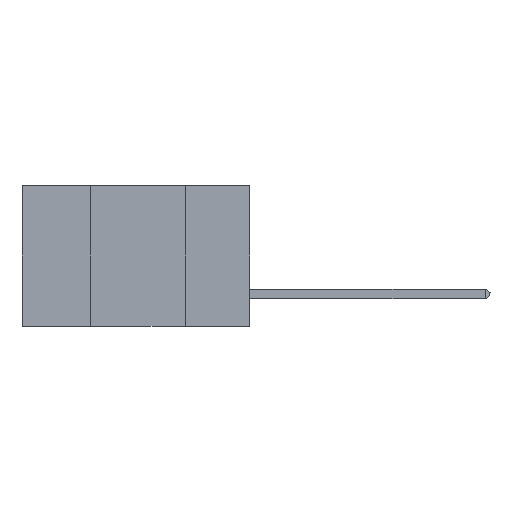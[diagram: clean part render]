
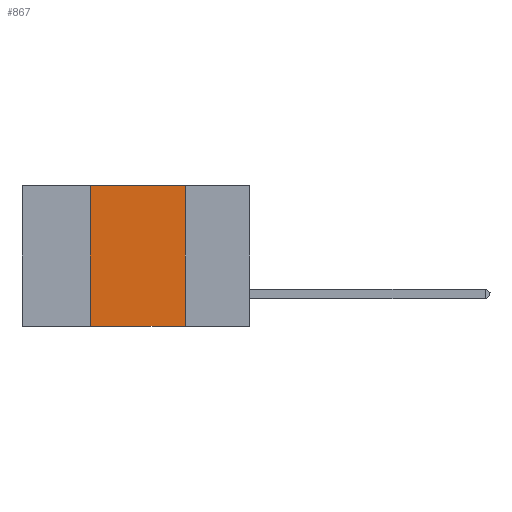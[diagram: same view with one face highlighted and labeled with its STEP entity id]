
A CAD part, left-side view. The second image highlights one B-rep face of the part: STEP entity #867.
In plain terms, the highlighted planar face has unit normal (-1, 0, 0).
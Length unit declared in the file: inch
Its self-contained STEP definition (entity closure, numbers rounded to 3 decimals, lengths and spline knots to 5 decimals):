
#100 = VECTOR ( 'NONE', #4592, 39.37008 ) ;
#669 = DIRECTION ( 'NONE',  ( 0., 0., -1. ) ) ;
#867 = ADVANCED_FACE ( 'NONE', ( #1939 ), #8767, .F. ) ;
#1110 = EDGE_CURVE ( 'NONE', #10636, #9905, #13705, .T. ) ;
#1291 = VERTEX_POINT ( 'NONE', #4663 ) ;
#1894 = ORIENTED_EDGE ( 'NONE', *, *, #5436, .F. ) ;
#1939 = FACE_OUTER_BOUND ( 'NONE', #13257, .T. ) ;
#3651 = CARTESIAN_POINT ( 'NONE',  ( 0., 0.17, 0. ) ) ;
#3675 = ORIENTED_EDGE ( 'NONE', *, *, #1110, .F. ) ;
#3711 = EDGE_CURVE ( 'NONE', #10761, #1291, #13244, .T. ) ;
#4373 = DIRECTION ( 'NONE',  ( 0., 0., -1. ) ) ;
#4592 = DIRECTION ( 'NONE',  ( 0., -1., 0. ) ) ;
#4663 = CARTESIAN_POINT ( 'NONE',  ( 0., 0.17, -0.37 ) ) ;
#5418 = DIRECTION ( 'NONE',  ( 1., 0., 0. ) ) ;
#5436 = EDGE_CURVE ( 'NONE', #9905, #10761, #8545, .T. ) ;
#5582 = ORIENTED_EDGE ( 'NONE', *, *, #3711, .F. ) ;
#5918 = VECTOR ( 'NONE', #12029, 39.37008 ) ;
#6578 = CARTESIAN_POINT ( 'NONE',  ( 0., 0.42, 0. ) ) ;
#6890 = LINE ( 'NONE', #13391, #100 ) ;
#7086 = VECTOR ( 'NONE', #14372, 39.37008 ) ;
#7927 = ORIENTED_EDGE ( 'NONE', *, *, #8289, .T. ) ;
#8289 = EDGE_CURVE ( 'NONE', #10636, #1291, #6890, .T. ) ;
#8545 = LINE ( 'NONE', #10694, #5918 ) ;
#8767 = PLANE ( 'NONE',  #14174 ) ;
#8982 = CARTESIAN_POINT ( 'NONE',  ( 0., 0.42, 0. ) ) ;
#9905 = VERTEX_POINT ( 'NONE', #8982 ) ;
#10473 = VECTOR ( 'NONE', #669, 39.37008 ) ;
#10636 = VERTEX_POINT ( 'NONE', #11184 ) ;
#10694 = CARTESIAN_POINT ( 'NONE',  ( 0., 0.6, 0. ) ) ;
#10761 = VERTEX_POINT ( 'NONE', #3651 ) ;
#11120 = CARTESIAN_POINT ( 'NONE',  ( 0., 0.6, 0. ) ) ;
#11184 = CARTESIAN_POINT ( 'NONE',  ( 0., 0.42, -0.37 ) ) ;
#12029 = DIRECTION ( 'NONE',  ( 0., -1., 0. ) ) ;
#13244 = LINE ( 'NONE', #13895, #10473 ) ;
#13257 = EDGE_LOOP ( 'NONE', ( #5582, #1894, #3675, #7927 ) ) ;
#13391 = CARTESIAN_POINT ( 'NONE',  ( 0., 0.6, -0.37 ) ) ;
#13705 = LINE ( 'NONE', #6578, #7086 ) ;
#13895 = CARTESIAN_POINT ( 'NONE',  ( 0., 0.17, 0. ) ) ;
#14174 = AXIS2_PLACEMENT_3D ( 'NONE', #11120, #5418, #4373 ) ;
#14372 = DIRECTION ( 'NONE',  ( 0., 0., 1. ) ) ;
